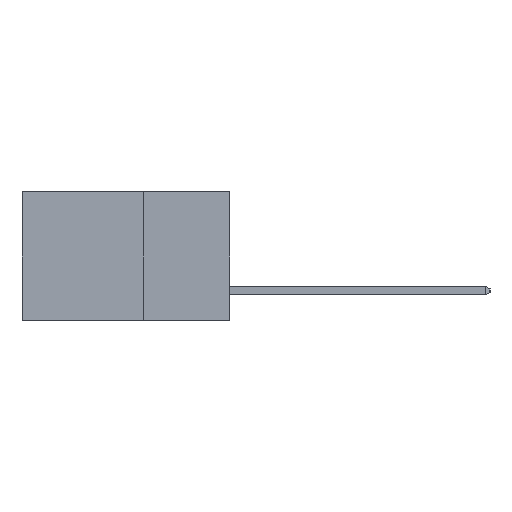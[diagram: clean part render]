
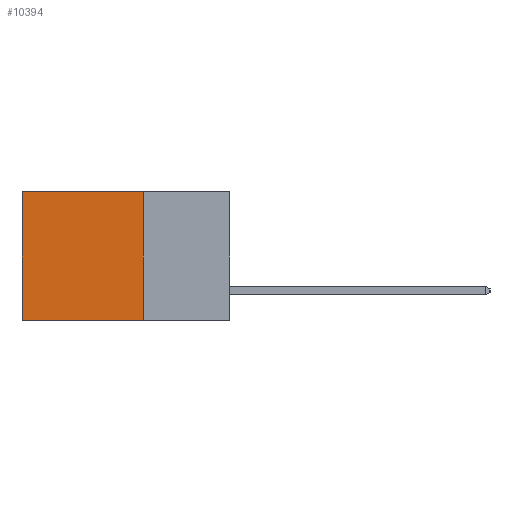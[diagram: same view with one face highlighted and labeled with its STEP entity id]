
A CAD part, left-side view. The second image highlights one B-rep face of the part: STEP entity #10394.
In plain terms, the highlighted planar face has unit normal (-1, 0, 0).
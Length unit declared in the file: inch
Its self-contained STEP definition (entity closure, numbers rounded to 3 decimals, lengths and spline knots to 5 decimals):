
#271 = EDGE_CURVE ( 'NONE', #11525, #11390, #6388, .T. ) ;
#1077 = CARTESIAN_POINT ( 'NONE',  ( 0.2615, 0.25, -0.37 ) ) ;
#1247 = VECTOR ( 'NONE', #2074, 39.37008 ) ;
#1492 = DIRECTION ( 'NONE',  ( 0., 1., 0. ) ) ;
#2074 = DIRECTION ( 'NONE',  ( 0., 1., 0. ) ) ;
#2317 = CARTESIAN_POINT ( 'NONE',  ( 0.2615, 0.25, 0. ) ) ;
#3238 = AXIS2_PLACEMENT_3D ( 'NONE', #3375, #6969, #11529 ) ;
#3375 = CARTESIAN_POINT ( 'NONE',  ( 0.2615, 0.25, -0.37 ) ) ;
#4313 = VECTOR ( 'NONE', #8985, 39.37008 ) ;
#5401 = CARTESIAN_POINT ( 'NONE',  ( 0.2615, 0.6, 0. ) ) ;
#5433 = FACE_OUTER_BOUND ( 'NONE', #9081, .T. ) ;
#5532 = VERTEX_POINT ( 'NONE', #7645 ) ;
#5855 = DIRECTION ( 'NONE',  ( 0., 0., -1. ) ) ;
#6388 = LINE ( 'NONE', #13996, #9416 ) ;
#6860 = VECTOR ( 'NONE', #5855, 39.37008 ) ;
#6969 = DIRECTION ( 'NONE',  ( 1., 0., 0. ) ) ;
#7374 = LINE ( 'NONE', #1077, #4313 ) ;
#7645 = CARTESIAN_POINT ( 'NONE',  ( 0.2615, 0.6, -0.37 ) ) ;
#7831 = CARTESIAN_POINT ( 'NONE',  ( 0.2615, 0.25, -0.37 ) ) ;
#8020 = PLANE ( 'NONE',  #3238 ) ;
#8797 = ORIENTED_EDGE ( 'NONE', *, *, #271, .T. ) ;
#8985 = DIRECTION ( 'NONE',  ( 0., 0., -1. ) ) ;
#9081 = EDGE_LOOP ( 'NONE', ( #11733, #13688, #13979, #8797 ) ) ;
#9416 = VECTOR ( 'NONE', #1492, 39.37008 ) ;
#10005 = EDGE_CURVE ( 'NONE', #11390, #5532, #12764, .T. ) ;
#10375 = LINE ( 'NONE', #7831, #1247 ) ;
#10394 = ADVANCED_FACE ( 'NONE', ( #5433 ), #8020, .F. ) ;
#11281 = VERTEX_POINT ( 'NONE', #13796 ) ;
#11390 = VERTEX_POINT ( 'NONE', #5401 ) ;
#11481 = EDGE_CURVE ( 'NONE', #11525, #11281, #7374, .T. ) ;
#11525 = VERTEX_POINT ( 'NONE', #2317 ) ;
#11529 = DIRECTION ( 'NONE',  ( 0., 0., -1. ) ) ;
#11733 = ORIENTED_EDGE ( 'NONE', *, *, #10005, .T. ) ;
#12196 = EDGE_CURVE ( 'NONE', #11281, #5532, #10375, .T. ) ;
#12764 = LINE ( 'NONE', #12811, #6860 ) ;
#12811 = CARTESIAN_POINT ( 'NONE',  ( 0.2615, 0.6, -0.37 ) ) ;
#13688 = ORIENTED_EDGE ( 'NONE', *, *, #12196, .F. ) ;
#13796 = CARTESIAN_POINT ( 'NONE',  ( 0.2615, 0.25, -0.37 ) ) ;
#13979 = ORIENTED_EDGE ( 'NONE', *, *, #11481, .F. ) ;
#13996 = CARTESIAN_POINT ( 'NONE',  ( 0.2615, 0.25, 0. ) ) ;
